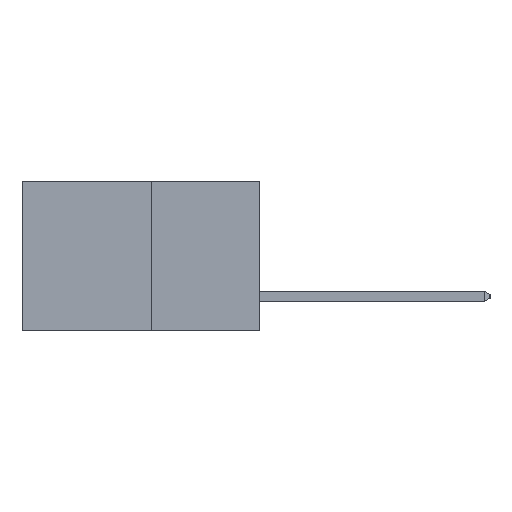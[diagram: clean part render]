
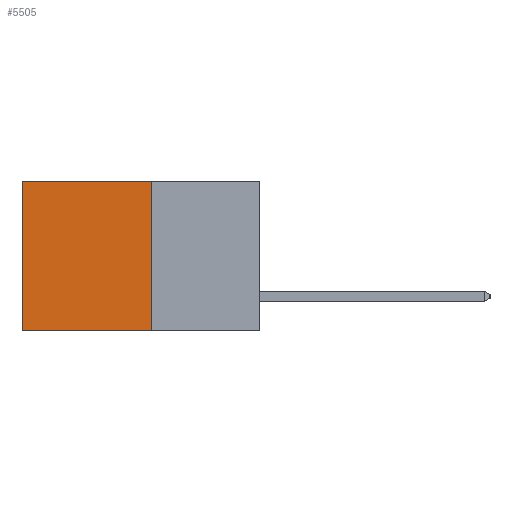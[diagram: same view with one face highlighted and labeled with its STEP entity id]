
A CAD part, left-side view. The second image highlights one B-rep face of the part: STEP entity #5505.
In plain terms, the highlighted planar face has unit normal (-1, 0, 0).
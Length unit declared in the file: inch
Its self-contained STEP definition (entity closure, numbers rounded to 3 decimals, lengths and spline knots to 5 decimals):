
#91 = ORIENTED_EDGE ( 'NONE', *, *, #5027, .F. ) ;
#446 = LINE ( 'NONE', #5368, #6339 ) ;
#801 = CARTESIAN_POINT ( 'NONE',  ( 0.277, 0.27, 0. ) ) ;
#859 = EDGE_LOOP ( 'NONE', ( #1748, #1583, #91, #4165 ) ) ;
#1482 = DIRECTION ( 'NONE',  ( 0., 0., -1. ) ) ;
#1583 = ORIENTED_EDGE ( 'NONE', *, *, #2977, .F. ) ;
#1748 = ORIENTED_EDGE ( 'NONE', *, *, #4600, .T. ) ;
#1811 = AXIS2_PLACEMENT_3D ( 'NONE', #5133, #7328, #2903 ) ;
#2191 = VERTEX_POINT ( 'NONE', #3289 ) ;
#2903 = DIRECTION ( 'NONE',  ( 0., 0., -1. ) ) ;
#2977 = EDGE_CURVE ( 'NONE', #7564, #2191, #446, .T. ) ;
#3289 = CARTESIAN_POINT ( 'NONE',  ( 0.277, 0.59, -0.37 ) ) ;
#3472 = VERTEX_POINT ( 'NONE', #5528 ) ;
#4145 = EDGE_CURVE ( 'NONE', #9216, #3472, #9530, .T. ) ;
#4165 = ORIENTED_EDGE ( 'NONE', *, *, #4145, .T. ) ;
#4229 = LINE ( 'NONE', #4830, #5964 ) ;
#4600 = EDGE_CURVE ( 'NONE', #3472, #2191, #4229, .T. ) ;
#4814 = LINE ( 'NONE', #9636, #5032 ) ;
#4830 = CARTESIAN_POINT ( 'NONE',  ( 0.277, 0.59, -0.37 ) ) ;
#5027 = EDGE_CURVE ( 'NONE', #9216, #7564, #4814, .T. ) ;
#5032 = VECTOR ( 'NONE', #1482, 39.37008 ) ;
#5133 = CARTESIAN_POINT ( 'NONE',  ( 0.277, 0.27, -0.37 ) ) ;
#5368 = CARTESIAN_POINT ( 'NONE',  ( 0.277, 0.27, -0.37 ) ) ;
#5505 = ADVANCED_FACE ( 'NONE', ( #5893 ), #9383, .F. ) ;
#5528 = CARTESIAN_POINT ( 'NONE',  ( 0.277, 0.59, 0. ) ) ;
#5752 = CARTESIAN_POINT ( 'NONE',  ( 0.277, 0.27, 0. ) ) ;
#5893 = FACE_OUTER_BOUND ( 'NONE', #859, .T. ) ;
#5964 = VECTOR ( 'NONE', #9115, 39.37008 ) ;
#6246 = CARTESIAN_POINT ( 'NONE',  ( 0.277, 0.27, -0.37 ) ) ;
#6339 = VECTOR ( 'NONE', #7572, 39.37008 ) ;
#6423 = VECTOR ( 'NONE', #7149, 39.37008 ) ;
#7149 = DIRECTION ( 'NONE',  ( 0., 1., 0. ) ) ;
#7328 = DIRECTION ( 'NONE',  ( 1., 0., 0. ) ) ;
#7564 = VERTEX_POINT ( 'NONE', #6246 ) ;
#7572 = DIRECTION ( 'NONE',  ( 0., 1., 0. ) ) ;
#9115 = DIRECTION ( 'NONE',  ( 0., 0., -1. ) ) ;
#9216 = VERTEX_POINT ( 'NONE', #801 ) ;
#9383 = PLANE ( 'NONE',  #1811 ) ;
#9530 = LINE ( 'NONE', #5752, #6423 ) ;
#9636 = CARTESIAN_POINT ( 'NONE',  ( 0.277, 0.27, -0.37 ) ) ;
